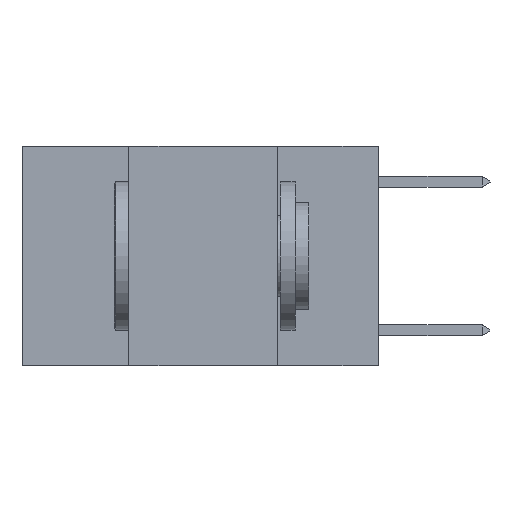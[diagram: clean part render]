
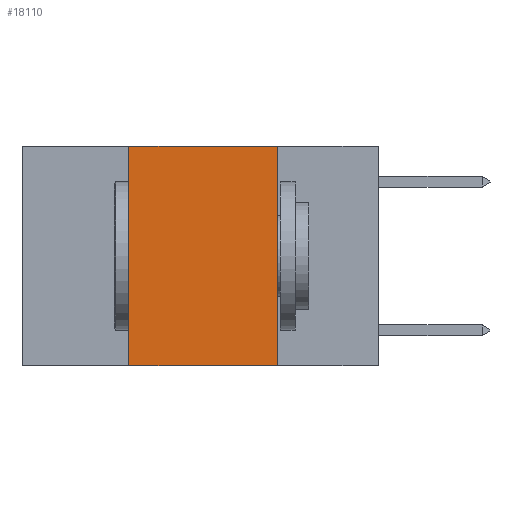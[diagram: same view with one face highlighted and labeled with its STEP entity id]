
A CAD part, left-side view. The second image highlights one B-rep face of the part: STEP entity #18110.
In plain terms, the highlighted planar face has unit normal (-1, 0, 0).
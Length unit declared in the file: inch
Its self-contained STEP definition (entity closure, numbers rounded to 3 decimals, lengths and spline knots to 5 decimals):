
#388 = AXIS2_PLACEMENT_3D ( 'NONE', #25126, #4194, #19011 ) ;
#1247 = EDGE_CURVE ( 'NONE', #11562, #16168, #7683, .T. ) ;
#4194 = DIRECTION ( 'NONE',  ( 1., 0., 0. ) ) ;
#4326 = CARTESIAN_POINT ( 'NONE',  ( 0., 0.6, 0. ) ) ;
#4358 = EDGE_LOOP ( 'NONE', ( #12629, #18774, #8265, #18443 ) ) ;
#5371 = FACE_OUTER_BOUND ( 'NONE', #4358, .T. ) ;
#5729 = VECTOR ( 'NONE', #13886, 39.37008 ) ;
#6844 = DIRECTION ( 'NONE',  ( 0., 0., 1. ) ) ;
#7519 = VERTEX_POINT ( 'NONE', #17941 ) ;
#7683 = LINE ( 'NONE', #19876, #12046 ) ;
#8265 = ORIENTED_EDGE ( 'NONE', *, *, #11461, .F. ) ;
#8468 = PLANE ( 'NONE',  #388 ) ;
#8778 = DIRECTION ( 'NONE',  ( 0., -1., 0. ) ) ;
#10108 = LINE ( 'NONE', #20092, #5729 ) ;
#10476 = VERTEX_POINT ( 'NONE', #22981 ) ;
#11461 = EDGE_CURVE ( 'NONE', #10476, #7519, #22923, .T. ) ;
#11562 = VERTEX_POINT ( 'NONE', #15650 ) ;
#12046 = VECTOR ( 'NONE', #25706, 39.37008 ) ;
#12629 = ORIENTED_EDGE ( 'NONE', *, *, #1247, .F. ) ;
#12742 = EDGE_CURVE ( 'NONE', #7519, #11562, #23857, .T. ) ;
#13886 = DIRECTION ( 'NONE',  ( 0., -1., 0. ) ) ;
#15650 = CARTESIAN_POINT ( 'NONE',  ( 0., 0.17, 0. ) ) ;
#16168 = VERTEX_POINT ( 'NONE', #24932 ) ;
#17213 = EDGE_CURVE ( 'NONE', #10476, #16168, #10108, .T. ) ;
#17727 = VECTOR ( 'NONE', #8778, 39.37008 ) ;
#17941 = CARTESIAN_POINT ( 'NONE',  ( 0., 0.42, 0. ) ) ;
#18110 = ADVANCED_FACE ( 'NONE', ( #5371 ), #8468, .F. ) ;
#18443 = ORIENTED_EDGE ( 'NONE', *, *, #17213, .T. ) ;
#18774 = ORIENTED_EDGE ( 'NONE', *, *, #12742, .F. ) ;
#19011 = DIRECTION ( 'NONE',  ( 0., 0., -1. ) ) ;
#19876 = CARTESIAN_POINT ( 'NONE',  ( 0., 0.17, 0. ) ) ;
#20092 = CARTESIAN_POINT ( 'NONE',  ( 0., 0.6, -0.37 ) ) ;
#21629 = VECTOR ( 'NONE', #6844, 39.37008 ) ;
#22923 = LINE ( 'NONE', #25589, #21629 ) ;
#22981 = CARTESIAN_POINT ( 'NONE',  ( 0., 0.42, -0.37 ) ) ;
#23857 = LINE ( 'NONE', #4326, #17727 ) ;
#24932 = CARTESIAN_POINT ( 'NONE',  ( 0., 0.17, -0.37 ) ) ;
#25126 = CARTESIAN_POINT ( 'NONE',  ( 0., 0.6, 0. ) ) ;
#25589 = CARTESIAN_POINT ( 'NONE',  ( 0., 0.42, 0. ) ) ;
#25706 = DIRECTION ( 'NONE',  ( 0., 0., -1. ) ) ;
